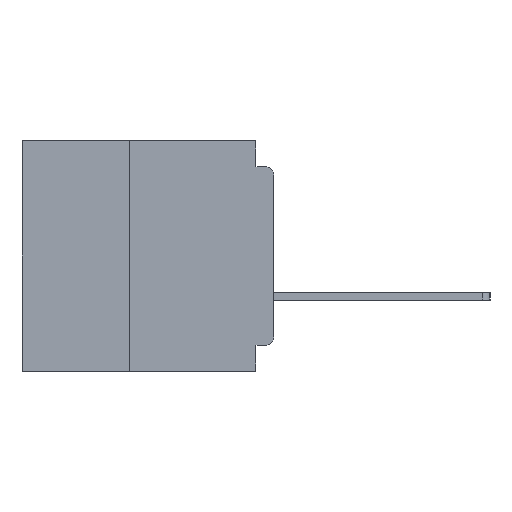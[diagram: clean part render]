
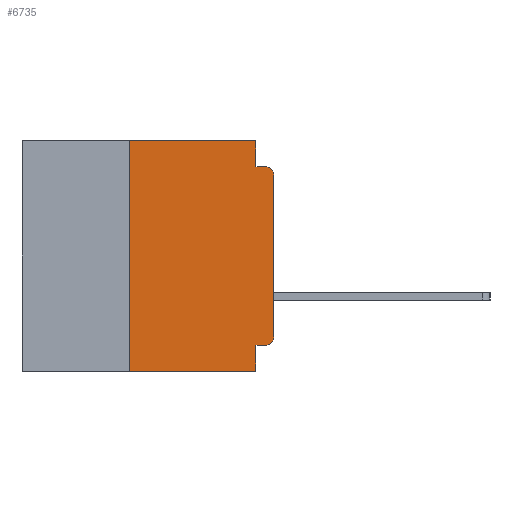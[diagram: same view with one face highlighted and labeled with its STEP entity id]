
A CAD part, left-side view. The second image highlights one B-rep face of the part: STEP entity #6735.
In plain terms, the highlighted planar face has unit normal (-1, 0, 0).
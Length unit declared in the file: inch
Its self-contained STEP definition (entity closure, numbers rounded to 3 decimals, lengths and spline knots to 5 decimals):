
#1111 = AXIS2_PLACEMENT_3D ( 'NONE', #24872, #55307, #29212 ) ;
#1767 = CARTESIAN_POINT ( 'NONE',  ( 0., 0., -0.06 ) ) ;
#1819 = VERTEX_POINT ( 'NONE', #45140 ) ;
#2048 = PLANE ( 'NONE',  #34020 ) ;
#3296 = EDGE_CURVE ( 'NONE', #19461, #27399, #16355, .T. ) ;
#3395 = CARTESIAN_POINT ( 'NONE',  ( 0., 0.031, -0.4 ) ) ;
#3549 = ORIENTED_EDGE ( 'NONE', *, *, #25523, .F. ) ;
#3940 = DIRECTION ( 'NONE',  ( 0., 0., 1. ) ) ;
#4372 = VERTEX_POINT ( 'NONE', #33131 ) ;
#5877 = VECTOR ( 'NONE', #29847, 39.37008 ) ;
#6735 = ADVANCED_FACE ( 'NONE', ( #18688 ), #2048, .F. ) ;
#6765 = DIRECTION ( 'NONE',  ( 0., -1., 0. ) ) ;
#9556 = CARTESIAN_POINT ( 'NONE',  ( 0., 0.031, -0.355 ) ) ;
#9873 = DIRECTION ( 'NONE',  ( -1., 0., 0. ) ) ;
#10926 = DIRECTION ( 'NONE',  ( 0., 0., -1. ) ) ;
#10976 = DIRECTION ( 'NONE',  ( 1., 0., 0. ) ) ;
#11396 = CARTESIAN_POINT ( 'NONE',  ( 0., 0.015, -0.045 ) ) ;
#11710 = LINE ( 'NONE', #24049, #46620 ) ;
#11741 = ORIENTED_EDGE ( 'NONE', *, *, #30437, .T. ) ;
#13107 = DIRECTION ( 'NONE',  ( 0., -1., 0. ) ) ;
#13278 = VECTOR ( 'NONE', #6765, 39.37008 ) ;
#13756 = EDGE_CURVE ( 'NONE', #4372, #20037, #29774, .T. ) ;
#14029 = VERTEX_POINT ( 'NONE', #1767 ) ;
#14330 = DIRECTION ( 'NONE',  ( 0., 0., 1. ) ) ;
#14747 = LINE ( 'NONE', #54732, #36600 ) ;
#15196 = ORIENTED_EDGE ( 'NONE', *, *, #3296, .F. ) ;
#15361 = VECTOR ( 'NONE', #13107, 39.37008 ) ;
#16355 = LINE ( 'NONE', #3395, #5877 ) ;
#18232 = CARTESIAN_POINT ( 'NONE',  ( 0., 0.031, -0.4 ) ) ;
#18554 = VERTEX_POINT ( 'NONE', #11396 ) ;
#18688 = FACE_OUTER_BOUND ( 'NONE', #45871, .T. ) ;
#19461 = VERTEX_POINT ( 'NONE', #9556 ) ;
#19847 = CARTESIAN_POINT ( 'NONE',  ( 0., 0.437, -0.4 ) ) ;
#20037 = VERTEX_POINT ( 'NONE', #22535 ) ;
#20986 = VECTOR ( 'NONE', #24248, 39.37008 ) ;
#22108 = EDGE_CURVE ( 'NONE', #14029, #18554, #47056, .T. ) ;
#22208 = CIRCLE ( 'NONE', #48875, 0.015 ) ;
#22535 = CARTESIAN_POINT ( 'NONE',  ( 0., 0.031, 0. ) ) ;
#23778 = EDGE_CURVE ( 'NONE', #20037, #43450, #14747, .T. ) ;
#24049 = CARTESIAN_POINT ( 'NONE',  ( 0., 0., -0.355 ) ) ;
#24248 = DIRECTION ( 'NONE',  ( 0., -1., 0. ) ) ;
#24872 = CARTESIAN_POINT ( 'NONE',  ( 0., 0.015, -0.06 ) ) ;
#25038 = LINE ( 'NONE', #37284, #13278 ) ;
#25057 = LINE ( 'NONE', #43455, #46775 ) ;
#25523 = EDGE_CURVE ( 'NONE', #32535, #19461, #11710, .T. ) ;
#27399 = VERTEX_POINT ( 'NONE', #18232 ) ;
#28473 = CARTESIAN_POINT ( 'NONE',  ( 0., 0.015, -0.355 ) ) ;
#28855 = EDGE_CURVE ( 'NONE', #43450, #18554, #25038, .T. ) ;
#29082 = VERTEX_POINT ( 'NONE', #43349 ) ;
#29212 = DIRECTION ( 'NONE',  ( 0., 0., -1. ) ) ;
#29774 = LINE ( 'NONE', #39290, #15361 ) ;
#29847 = DIRECTION ( 'NONE',  ( 0., 0., -1. ) ) ;
#30437 = EDGE_CURVE ( 'NONE', #32535, #1819, #22208, .T. ) ;
#30744 = ORIENTED_EDGE ( 'NONE', *, *, #50511, .F. ) ;
#32535 = VERTEX_POINT ( 'NONE', #28473 ) ;
#32877 = CARTESIAN_POINT ( 'NONE',  ( 0., 0.437, 0. ) ) ;
#33131 = CARTESIAN_POINT ( 'NONE',  ( 0., 0.25, 0. ) ) ;
#33676 = ORIENTED_EDGE ( 'NONE', *, *, #36293, .T. ) ;
#34020 = AXIS2_PLACEMENT_3D ( 'NONE', #32877, #10976, #41594 ) ;
#35635 = VECTOR ( 'NONE', #14330, 39.37008 ) ;
#36093 = ORIENTED_EDGE ( 'NONE', *, *, #13756, .F. ) ;
#36154 = CARTESIAN_POINT ( 'NONE',  ( 0., 0.015, -0.34 ) ) ;
#36293 = EDGE_CURVE ( 'NONE', #29082, #27399, #44073, .T. ) ;
#36600 = VECTOR ( 'NONE', #10926, 39.37008 ) ;
#37284 = CARTESIAN_POINT ( 'NONE',  ( 0., 0., -0.045 ) ) ;
#38436 = ORIENTED_EDGE ( 'NONE', *, *, #22108, .T. ) ;
#39290 = CARTESIAN_POINT ( 'NONE',  ( 0., 0.437, 0. ) ) ;
#40495 = DIRECTION ( 'NONE',  ( 0., 0., -1. ) ) ;
#41594 = DIRECTION ( 'NONE',  ( 0., 0., -1. ) ) ;
#43349 = CARTESIAN_POINT ( 'NONE',  ( 0., 0.25, -0.4 ) ) ;
#43450 = VERTEX_POINT ( 'NONE', #49444 ) ;
#43455 = CARTESIAN_POINT ( 'NONE',  ( 0., 0.25, -0.4 ) ) ;
#44073 = LINE ( 'NONE', #19847, #20986 ) ;
#44182 = ORIENTED_EDGE ( 'NONE', *, *, #52436, .T. ) ;
#45140 = CARTESIAN_POINT ( 'NONE',  ( 0., 0., -0.34 ) ) ;
#45871 = EDGE_LOOP ( 'NONE', ( #44182, #38436, #54797, #48000, #36093, #30744, #33676, #15196, #3549, #11741 ) ) ;
#46620 = VECTOR ( 'NONE', #50097, 39.37008 ) ;
#46775 = VECTOR ( 'NONE', #3940, 39.37008 ) ;
#47056 = CIRCLE ( 'NONE', #1111, 0.015 ) ;
#47246 = LINE ( 'NONE', #53474, #35635 ) ;
#48000 = ORIENTED_EDGE ( 'NONE', *, *, #23778, .F. ) ;
#48875 = AXIS2_PLACEMENT_3D ( 'NONE', #36154, #9873, #40495 ) ;
#49444 = CARTESIAN_POINT ( 'NONE',  ( 0., 0.031, -0.045 ) ) ;
#50097 = DIRECTION ( 'NONE',  ( 0., 1., 0. ) ) ;
#50511 = EDGE_CURVE ( 'NONE', #29082, #4372, #25057, .T. ) ;
#52436 = EDGE_CURVE ( 'NONE', #1819, #14029, #47246, .T. ) ;
#53474 = CARTESIAN_POINT ( 'NONE',  ( 0., 0., 0. ) ) ;
#54732 = CARTESIAN_POINT ( 'NONE',  ( 0., 0.031, 0. ) ) ;
#54797 = ORIENTED_EDGE ( 'NONE', *, *, #28855, .F. ) ;
#55307 = DIRECTION ( 'NONE',  ( -1., 0., 0. ) ) ;
